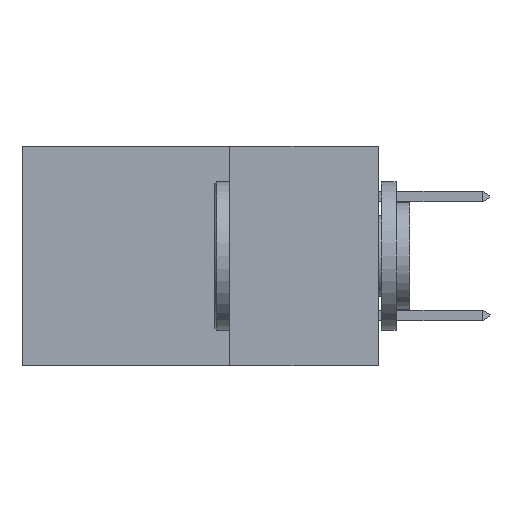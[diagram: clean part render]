
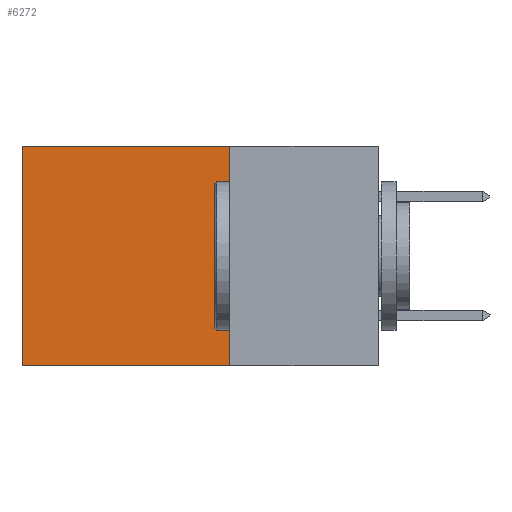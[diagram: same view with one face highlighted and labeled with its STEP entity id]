
A CAD part, left-side view. The second image highlights one B-rep face of the part: STEP entity #6272.
In plain terms, the highlighted planar face has unit normal (-1, 0, 0).
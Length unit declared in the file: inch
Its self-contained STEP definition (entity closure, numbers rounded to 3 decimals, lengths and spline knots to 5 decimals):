
#96 = CARTESIAN_POINT ( 'NONE',  ( 0.298, 0.25, -0.37 ) ) ;
#557 = DIRECTION ( 'NONE',  ( 0., 0., -1. ) ) ;
#761 = VERTEX_POINT ( 'NONE', #8182 ) ;
#877 = VERTEX_POINT ( 'NONE', #96 ) ;
#915 = DIRECTION ( 'NONE',  ( 0., 1., 0. ) ) ;
#1575 = FACE_OUTER_BOUND ( 'NONE', #3955, .T. ) ;
#1706 = AXIS2_PLACEMENT_3D ( 'NONE', #11561, #6032, #557 ) ;
#2191 = CARTESIAN_POINT ( 'NONE',  ( 0.298, 0.25, -0.37 ) ) ;
#2870 = CARTESIAN_POINT ( 'NONE',  ( 0.298, 0.6, 0. ) ) ;
#3635 = LINE ( 'NONE', #2191, #11966 ) ;
#3955 = EDGE_LOOP ( 'NONE', ( #5468, #8201, #11627, #10983 ) ) ;
#3970 = CARTESIAN_POINT ( 'NONE',  ( 0.298, 0.25, 0. ) ) ;
#4063 = DIRECTION ( 'NONE',  ( 0., 1., 0. ) ) ;
#4693 = VECTOR ( 'NONE', #5027, 39.37008 ) ;
#5027 = DIRECTION ( 'NONE',  ( 0., 0., -1. ) ) ;
#5468 = ORIENTED_EDGE ( 'NONE', *, *, #6547, .T. ) ;
#5748 = VERTEX_POINT ( 'NONE', #5757 ) ;
#5757 = CARTESIAN_POINT ( 'NONE',  ( 0.298, 0.6, 0. ) ) ;
#5924 = CARTESIAN_POINT ( 'NONE',  ( 0.298, 0.25, 0. ) ) ;
#6032 = DIRECTION ( 'NONE',  ( 1., 0., 0. ) ) ;
#6272 = ADVANCED_FACE ( 'NONE', ( #1575 ), #11600, .F. ) ;
#6547 = EDGE_CURVE ( 'NONE', #5748, #761, #9258, .T. ) ;
#6561 = DIRECTION ( 'NONE',  ( 0., 0., -1. ) ) ;
#7954 = VECTOR ( 'NONE', #6561, 39.37008 ) ;
#8182 = CARTESIAN_POINT ( 'NONE',  ( 0.298, 0.6, -0.37 ) ) ;
#8201 = ORIENTED_EDGE ( 'NONE', *, *, #9027, .F. ) ;
#8392 = VERTEX_POINT ( 'NONE', #3970 ) ;
#8441 = EDGE_CURVE ( 'NONE', #8392, #877, #9823, .T. ) ;
#9027 = EDGE_CURVE ( 'NONE', #877, #761, #3635, .T. ) ;
#9258 = LINE ( 'NONE', #2870, #7954 ) ;
#9267 = CARTESIAN_POINT ( 'NONE',  ( 0.298, 0.25, 0. ) ) ;
#9823 = LINE ( 'NONE', #5924, #4693 ) ;
#10983 = ORIENTED_EDGE ( 'NONE', *, *, #11951, .T. ) ;
#11181 = LINE ( 'NONE', #9267, #11890 ) ;
#11561 = CARTESIAN_POINT ( 'NONE',  ( 0.298, 0.25, 0. ) ) ;
#11600 = PLANE ( 'NONE',  #1706 ) ;
#11627 = ORIENTED_EDGE ( 'NONE', *, *, #8441, .F. ) ;
#11890 = VECTOR ( 'NONE', #915, 39.37008 ) ;
#11951 = EDGE_CURVE ( 'NONE', #8392, #5748, #11181, .T. ) ;
#11966 = VECTOR ( 'NONE', #4063, 39.37008 ) ;
